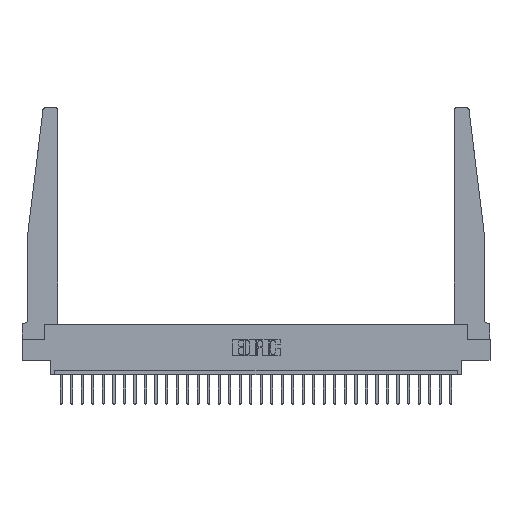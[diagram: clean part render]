
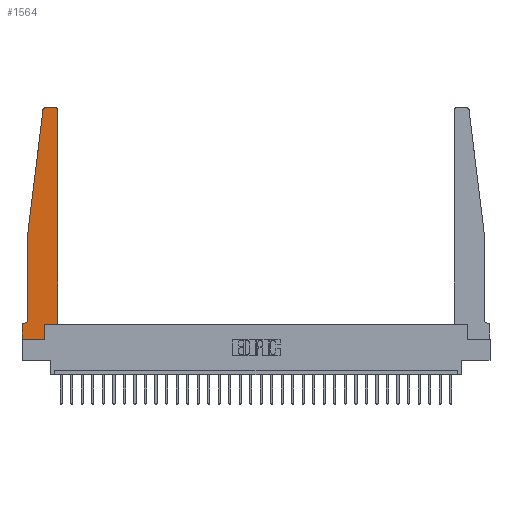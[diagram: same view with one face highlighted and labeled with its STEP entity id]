
A CAD part, top view. The second image highlights one B-rep face of the part: STEP entity #1564.
In plain terms, the highlighted planar face has unit normal (0, 0, 1).
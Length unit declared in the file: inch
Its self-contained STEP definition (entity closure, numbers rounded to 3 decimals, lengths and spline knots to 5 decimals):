
#493 = CARTESIAN_POINT ( 'NONE',  ( 0.2605, 0.18, 0.37 ) ) ;
#659 = VERTEX_POINT ( 'NONE', #23495 ) ;
#1564 = ADVANCED_FACE ( 'NONE', ( #28996 ), #24250, .T. ) ;
#2778 = DIRECTION ( 'NONE',  ( 1., 0., 0. ) ) ;
#3067 = DIRECTION ( 'NONE',  ( 0., -1., 0. ) ) ;
#3711 = ORIENTED_EDGE ( 'NONE', *, *, #6513, .T. ) ;
#3787 = EDGE_CURVE ( 'NONE', #8103, #4957, #27013, .T. ) ;
#3906 = CARTESIAN_POINT ( 'NONE',  ( 0.065, 0.1875, 0.37 ) ) ;
#4594 = DIRECTION ( 'NONE',  ( 1., 0., 0. ) ) ;
#4620 = CARTESIAN_POINT ( 'NONE',  ( 0.2605, 0., 0.37 ) ) ;
#4957 = VERTEX_POINT ( 'NONE', #27172 ) ;
#5561 = CARTESIAN_POINT ( 'NONE',  ( 0.395, 2.75, 0.37 ) ) ;
#5816 = EDGE_CURVE ( 'NONE', #25033, #11773, #28755, .T. ) ;
#6189 = DIRECTION ( 'NONE',  ( -1., 0., 0. ) ) ;
#6501 = DIRECTION ( 'NONE',  ( 1., 0., 0. ) ) ;
#6513 = EDGE_CURVE ( 'NONE', #15994, #659, #11053, .T. ) ;
#6956 = ORIENTED_EDGE ( 'NONE', *, *, #14419, .T. ) ;
#7502 = ORIENTED_EDGE ( 'NONE', *, *, #17848, .T. ) ;
#8046 = DIRECTION ( 'NONE',  ( 1., 0., 0. ) ) ;
#8086 = AXIS2_PLACEMENT_3D ( 'NONE', #18796, #25809, #23156 ) ;
#8103 = VERTEX_POINT ( 'NONE', #5561 ) ;
#8359 = CARTESIAN_POINT ( 'NONE',  ( 0.065, 1.25, 0.37 ) ) ;
#8426 = LINE ( 'NONE', #28817, #26723 ) ;
#8444 = VECTOR ( 'NONE', #12972, 39.37008 ) ;
#8548 = DIRECTION ( 'NONE',  ( 0., -1., 0. ) ) ;
#8574 = CIRCLE ( 'NONE', #8086, 0.05 ) ;
#9378 = VECTOR ( 'NONE', #8548, 39.37008 ) ;
#10576 = EDGE_CURVE ( 'NONE', #12613, #15994, #8574, .T. ) ;
#10725 = VECTOR ( 'NONE', #6189, 39.37008 ) ;
#10774 = LINE ( 'NONE', #28934, #9378 ) ;
#11053 = LINE ( 'NONE', #3906, #18346 ) ;
#11308 = EDGE_CURVE ( 'NONE', #28604, #25907, #21232, .T. ) ;
#11432 = VECTOR ( 'NONE', #12436, 39.37008 ) ;
#11673 = CARTESIAN_POINT ( 'NONE',  ( 0.425, 2.72, 0.37 ) ) ;
#11773 = VERTEX_POINT ( 'NONE', #16715 ) ;
#12077 = EDGE_LOOP ( 'NONE', ( #23254, #7502, #26051, #26565, #25164, #3711, #6956, #13341, #26913, #20783, #29226, #19469 ) ) ;
#12434 = VECTOR ( 'NONE', #3067, 39.37008 ) ;
#12436 = DIRECTION ( 'NONE',  ( 0., 1., 0. ) ) ;
#12613 = VERTEX_POINT ( 'NONE', #25743 ) ;
#12912 = DIRECTION ( 'NONE',  ( 0., 0., 1. ) ) ;
#12972 = DIRECTION ( 'NONE',  ( -0.122, -0.992, 0. ) ) ;
#13321 = CARTESIAN_POINT ( 'NONE',  ( 0.25, 2.75, 0.37 ) ) ;
#13341 = ORIENTED_EDGE ( 'NONE', *, *, #18645, .T. ) ;
#13926 = CARTESIAN_POINT ( 'NONE',  ( 0.425, 0.18, 0.37 ) ) ;
#14067 = DIRECTION ( 'NONE',  ( 0., 1., 0. ) ) ;
#14406 = EDGE_CURVE ( 'NONE', #21730, #8103, #23413, .T. ) ;
#14419 = EDGE_CURVE ( 'NONE', #659, #21431, #23500, .T. ) ;
#15994 = VERTEX_POINT ( 'NONE', #24461 ) ;
#16052 = DIRECTION ( 'NONE',  ( 0., 0., 1. ) ) ;
#16715 = CARTESIAN_POINT ( 'NONE',  ( 0.065, 1.25, 0.37 ) ) ;
#17631 = CIRCLE ( 'NONE', #21460, 0.03 ) ;
#17756 = VECTOR ( 'NONE', #8046, 39.37008 ) ;
#17848 = EDGE_CURVE ( 'NONE', #4957, #25033, #17631, .T. ) ;
#18128 = AXIS2_PLACEMENT_3D ( 'NONE', #25423, #20961, #2778 ) ;
#18203 = VECTOR ( 'NONE', #14067, 39.37008 ) ;
#18346 = VECTOR ( 'NONE', #22367, 39.37008 ) ;
#18396 = CARTESIAN_POINT ( 'NONE',  ( 0., 0., 0.37 ) ) ;
#18645 = EDGE_CURVE ( 'NONE', #21431, #28604, #8426, .T. ) ;
#18796 = CARTESIAN_POINT ( 'NONE',  ( 0.015, 0.2375, 0.37 ) ) ;
#19022 = CARTESIAN_POINT ( 'NONE',  ( 0.24675, 2.72367, 0.37 ) ) ;
#19469 = ORIENTED_EDGE ( 'NONE', *, *, #14406, .T. ) ;
#20008 = EDGE_CURVE ( 'NONE', #21588, #21730, #20778, .T. ) ;
#20778 = LINE ( 'NONE', #13926, #18203 ) ;
#20783 = ORIENTED_EDGE ( 'NONE', *, *, #22350, .T. ) ;
#20961 = DIRECTION ( 'NONE',  ( 0., 0., 1. ) ) ;
#21232 = LINE ( 'NONE', #25845, #11432 ) ;
#21431 = VERTEX_POINT ( 'NONE', #25440 ) ;
#21460 = AXIS2_PLACEMENT_3D ( 'NONE', #25004, #16052, #4594 ) ;
#21588 = VERTEX_POINT ( 'NONE', #29241 ) ;
#21730 = VERTEX_POINT ( 'NONE', #11673 ) ;
#21886 = CARTESIAN_POINT ( 'NONE',  ( 0.425, 0.18, 0.37 ) ) ;
#22169 = LINE ( 'NONE', #21886, #17756 ) ;
#22350 = EDGE_CURVE ( 'NONE', #25907, #21588, #22169, .T. ) ;
#22367 = DIRECTION ( 'NONE',  ( -1., 0., 0. ) ) ;
#23156 = DIRECTION ( 'NONE',  ( -1., 0., 0. ) ) ;
#23254 = ORIENTED_EDGE ( 'NONE', *, *, #3787, .T. ) ;
#23413 = CIRCLE ( 'NONE', #18128, 0.03 ) ;
#23495 = CARTESIAN_POINT ( 'NONE',  ( 0., 0.1875, 0.37 ) ) ;
#23500 = LINE ( 'NONE', #18396, #12434 ) ;
#24250 = PLANE ( 'NONE',  #25835 ) ;
#24461 = CARTESIAN_POINT ( 'NONE',  ( 0.015, 0.1875, 0.37 ) ) ;
#25004 = CARTESIAN_POINT ( 'NONE',  ( 0.27653, 2.72, 0.37 ) ) ;
#25033 = VERTEX_POINT ( 'NONE', #19022 ) ;
#25164 = ORIENTED_EDGE ( 'NONE', *, *, #10576, .T. ) ;
#25423 = CARTESIAN_POINT ( 'NONE',  ( 0.395, 2.72, 0.37 ) ) ;
#25440 = CARTESIAN_POINT ( 'NONE',  ( 0., 0., 0.37 ) ) ;
#25743 = CARTESIAN_POINT ( 'NONE',  ( 0.065, 0.2375, 0.37 ) ) ;
#25809 = DIRECTION ( 'NONE',  ( 0., 0., -1. ) ) ;
#25835 = AXIS2_PLACEMENT_3D ( 'NONE', #26890, #12912, #6501 ) ;
#25845 = CARTESIAN_POINT ( 'NONE',  ( 0.2605, 0.18, 0.37 ) ) ;
#25907 = VERTEX_POINT ( 'NONE', #493 ) ;
#26051 = ORIENTED_EDGE ( 'NONE', *, *, #5816, .T. ) ;
#26184 = EDGE_CURVE ( 'NONE', #11773, #12613, #10774, .T. ) ;
#26565 = ORIENTED_EDGE ( 'NONE', *, *, #26184, .T. ) ;
#26723 = VECTOR ( 'NONE', #28678, 39.37008 ) ;
#26890 = CARTESIAN_POINT ( 'NONE',  ( 0., 0.1875, 0.37 ) ) ;
#26913 = ORIENTED_EDGE ( 'NONE', *, *, #11308, .T. ) ;
#27013 = LINE ( 'NONE', #13321, #10725 ) ;
#27172 = CARTESIAN_POINT ( 'NONE',  ( 0.27653, 2.75, 0.37 ) ) ;
#28604 = VERTEX_POINT ( 'NONE', #4620 ) ;
#28678 = DIRECTION ( 'NONE',  ( 1., 0., 0. ) ) ;
#28755 = LINE ( 'NONE', #8359, #8444 ) ;
#28817 = CARTESIAN_POINT ( 'NONE',  ( 0., 0., 0.37 ) ) ;
#28934 = CARTESIAN_POINT ( 'NONE',  ( 0.065, 1.25, 0.37 ) ) ;
#28996 = FACE_OUTER_BOUND ( 'NONE', #12077, .T. ) ;
#29226 = ORIENTED_EDGE ( 'NONE', *, *, #20008, .T. ) ;
#29241 = CARTESIAN_POINT ( 'NONE',  ( 0.425, 0.18, 0.37 ) ) ;
